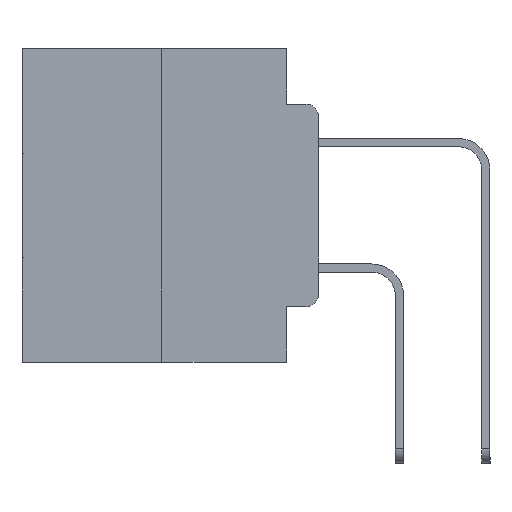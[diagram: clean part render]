
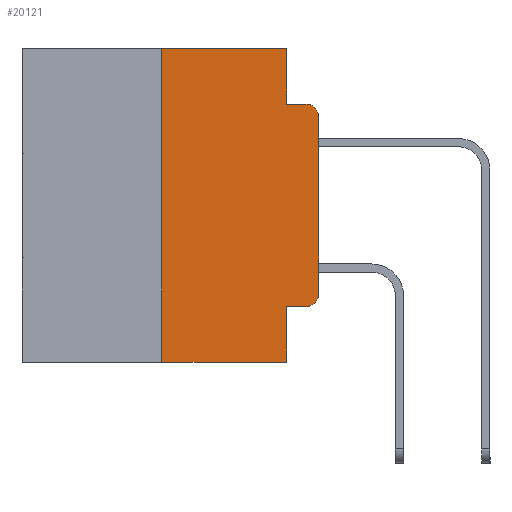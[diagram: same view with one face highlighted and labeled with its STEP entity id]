
A CAD part, left-side view. The second image highlights one B-rep face of the part: STEP entity #20121.
In plain terms, the highlighted planar face has unit normal (-1, 0, 0).
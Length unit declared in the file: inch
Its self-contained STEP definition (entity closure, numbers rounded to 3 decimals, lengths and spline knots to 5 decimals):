
#20 = CARTESIAN_POINT ( 'NONE',  ( 0., 0.051, -0.4115 ) ) ;
#349 = CARTESIAN_POINT ( 'NONE',  ( 0., 0.25, 0. ) ) ;
#836 = DIRECTION ( 'NONE',  ( 0., -1., 0. ) ) ;
#929 = EDGE_LOOP ( 'NONE', ( #27254, #12314, #8236, #26913, #28355, #18224, #1576, #14179, #4660, #6134 ) ) ;
#1335 = CARTESIAN_POINT ( 'NONE',  ( 0., 0.473, 0. ) ) ;
#1576 = ORIENTED_EDGE ( 'NONE', *, *, #12689, .T. ) ;
#1886 = AXIS2_PLACEMENT_3D ( 'NONE', #6635, #23037, #9018 ) ;
#2468 = CARTESIAN_POINT ( 'NONE',  ( 0., 0.25, 0. ) ) ;
#3152 = LINE ( 'NONE', #28203, #8702 ) ;
#3853 = VECTOR ( 'NONE', #11260, 39.37008 ) ;
#4660 = ORIENTED_EDGE ( 'NONE', *, *, #10698, .T. ) ;
#5397 = VECTOR ( 'NONE', #16602, 39.37008 ) ;
#5960 = CARTESIAN_POINT ( 'NONE',  ( 0., 0.25, -0.5 ) ) ;
#6134 = ORIENTED_EDGE ( 'NONE', *, *, #9139, .T. ) ;
#6635 = CARTESIAN_POINT ( 'NONE',  ( 0., 0.02, -0.3915 ) ) ;
#7462 = VERTEX_POINT ( 'NONE', #27988 ) ;
#7889 = DIRECTION ( 'NONE',  ( 0., 0., -1. ) ) ;
#7969 = VECTOR ( 'NONE', #29857, 39.37008 ) ;
#8236 = ORIENTED_EDGE ( 'NONE', *, *, #21673, .F. ) ;
#8567 = CIRCLE ( 'NONE', #15408, 0.02 ) ;
#8702 = VECTOR ( 'NONE', #9622, 39.37008 ) ;
#9018 = DIRECTION ( 'NONE',  ( 0., 0., -1. ) ) ;
#9139 = EDGE_CURVE ( 'NONE', #7462, #23144, #27823, .T. ) ;
#9622 = DIRECTION ( 'NONE',  ( 0., 0., -1. ) ) ;
#9710 = LINE ( 'NONE', #349, #22898 ) ;
#10698 = EDGE_CURVE ( 'NONE', #28517, #7462, #16478, .T. ) ;
#10700 = CARTESIAN_POINT ( 'NONE',  ( 0., 0.051, -0.5 ) ) ;
#10809 = CARTESIAN_POINT ( 'NONE',  ( 0., 0., -0.1085 ) ) ;
#10888 = DIRECTION ( 'NONE',  ( 0., -1., 0. ) ) ;
#11086 = CARTESIAN_POINT ( 'NONE',  ( 0., 0.02, -0.1085 ) ) ;
#11260 = DIRECTION ( 'NONE',  ( 0., 0., -1. ) ) ;
#12285 = EDGE_CURVE ( 'NONE', #28517, #29707, #22593, .T. ) ;
#12314 = ORIENTED_EDGE ( 'NONE', *, *, #24808, .T. ) ;
#12676 = CARTESIAN_POINT ( 'NONE',  ( 0., 0.473, -0.5 ) ) ;
#12689 = EDGE_CURVE ( 'NONE', #19099, #29707, #13084, .T. ) ;
#13084 = LINE ( 'NONE', #12676, #18585 ) ;
#13461 = DIRECTION ( 'NONE',  ( 0., 0., -1. ) ) ;
#13877 = EDGE_CURVE ( 'NONE', #19099, #24224, #9710, .T. ) ;
#14179 = ORIENTED_EDGE ( 'NONE', *, *, #12285, .F. ) ;
#14581 = DIRECTION ( 'NONE',  ( 0., 0., 1. ) ) ;
#14777 = VERTEX_POINT ( 'NONE', #10809 ) ;
#15183 = VECTOR ( 'NONE', #10888, 39.37008 ) ;
#15241 = VERTEX_POINT ( 'NONE', #26422 ) ;
#15408 = AXIS2_PLACEMENT_3D ( 'NONE', #11086, #27408, #13461 ) ;
#15967 = CARTESIAN_POINT ( 'NONE',  ( 0., 0., 0. ) ) ;
#16274 = CARTESIAN_POINT ( 'NONE',  ( 0., 0.051, -0.0885 ) ) ;
#16478 = LINE ( 'NONE', #20, #5397 ) ;
#16602 = DIRECTION ( 'NONE',  ( 0., -1., 0. ) ) ;
#18224 = ORIENTED_EDGE ( 'NONE', *, *, #13877, .F. ) ;
#18335 = VERTEX_POINT ( 'NONE', #29708 ) ;
#18584 = EDGE_CURVE ( 'NONE', #18335, #27989, #3152, .T. ) ;
#18585 = VECTOR ( 'NONE', #836, 39.37008 ) ;
#19099 = VERTEX_POINT ( 'NONE', #5960 ) ;
#19468 = CARTESIAN_POINT ( 'NONE',  ( 0., 0.473, 0. ) ) ;
#19566 = PLANE ( 'NONE',  #27794 ) ;
#19615 = CARTESIAN_POINT ( 'NONE',  ( 0., 0., -0.3915 ) ) ;
#20070 = LINE ( 'NONE', #27719, #25563 ) ;
#20121 = ADVANCED_FACE ( 'NONE', ( #22000 ), #19566, .F. ) ;
#21369 = LINE ( 'NONE', #1335, #15183 ) ;
#21673 = EDGE_CURVE ( 'NONE', #27989, #15241, #20070, .T. ) ;
#21903 = DIRECTION ( 'NONE',  ( 1., 0., 0. ) ) ;
#22000 = FACE_OUTER_BOUND ( 'NONE', #929, .T. ) ;
#22593 = LINE ( 'NONE', #29681, #3853 ) ;
#22898 = VECTOR ( 'NONE', #14581, 39.37008 ) ;
#23037 = DIRECTION ( 'NONE',  ( -1., 0., 0. ) ) ;
#23054 = DIRECTION ( 'NONE',  ( 0., -1., 0. ) ) ;
#23144 = VERTEX_POINT ( 'NONE', #19615 ) ;
#24224 = VERTEX_POINT ( 'NONE', #2468 ) ;
#24808 = EDGE_CURVE ( 'NONE', #14777, #15241, #8567, .T. ) ;
#25205 = CARTESIAN_POINT ( 'NONE',  ( 0., 0.051, -0.4115 ) ) ;
#25563 = VECTOR ( 'NONE', #23054, 39.37008 ) ;
#25916 = LINE ( 'NONE', #15967, #7969 ) ;
#26422 = CARTESIAN_POINT ( 'NONE',  ( 0., 0.02, -0.0885 ) ) ;
#26913 = ORIENTED_EDGE ( 'NONE', *, *, #18584, .F. ) ;
#27254 = ORIENTED_EDGE ( 'NONE', *, *, #27905, .T. ) ;
#27408 = DIRECTION ( 'NONE',  ( -1., 0., 0. ) ) ;
#27719 = CARTESIAN_POINT ( 'NONE',  ( 0., 0.051, -0.0885 ) ) ;
#27794 = AXIS2_PLACEMENT_3D ( 'NONE', #19468, #21903, #7889 ) ;
#27823 = CIRCLE ( 'NONE', #1886, 0.02 ) ;
#27905 = EDGE_CURVE ( 'NONE', #23144, #14777, #25916, .T. ) ;
#27988 = CARTESIAN_POINT ( 'NONE',  ( 0., 0.02, -0.4115 ) ) ;
#27989 = VERTEX_POINT ( 'NONE', #16274 ) ;
#28203 = CARTESIAN_POINT ( 'NONE',  ( 0., 0.051, 0. ) ) ;
#28355 = ORIENTED_EDGE ( 'NONE', *, *, #30237, .F. ) ;
#28517 = VERTEX_POINT ( 'NONE', #25205 ) ;
#29681 = CARTESIAN_POINT ( 'NONE',  ( 0., 0.051, 0. ) ) ;
#29707 = VERTEX_POINT ( 'NONE', #10700 ) ;
#29708 = CARTESIAN_POINT ( 'NONE',  ( 0., 0.051, 0. ) ) ;
#29857 = DIRECTION ( 'NONE',  ( 0., 0., 1. ) ) ;
#30237 = EDGE_CURVE ( 'NONE', #24224, #18335, #21369, .T. ) ;
